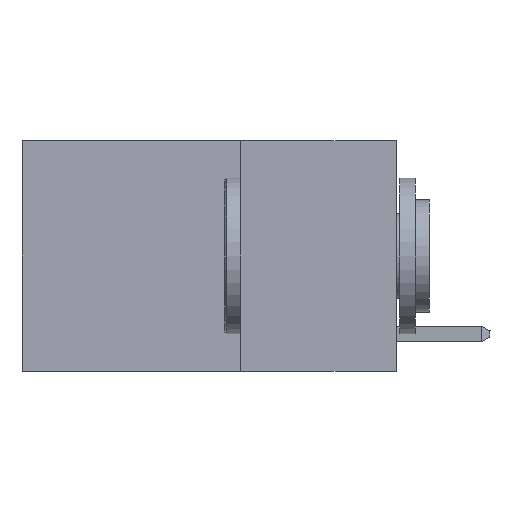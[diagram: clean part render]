
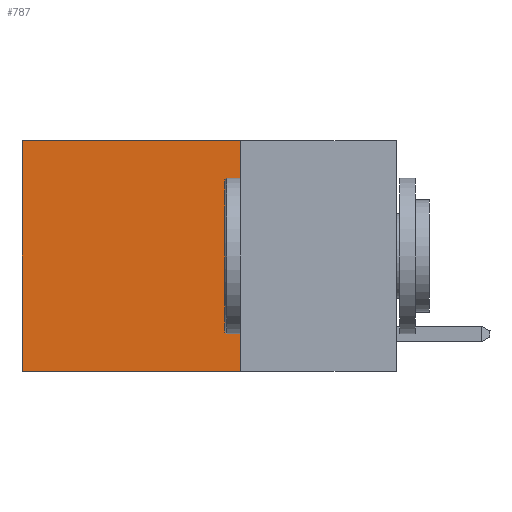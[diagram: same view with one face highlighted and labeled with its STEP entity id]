
A CAD part, left-side view. The second image highlights one B-rep face of the part: STEP entity #787.
In plain terms, the highlighted planar face has unit normal (-1, 0, 0).
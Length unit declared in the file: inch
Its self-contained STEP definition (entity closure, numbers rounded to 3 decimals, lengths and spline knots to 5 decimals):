
#426 = VERTEX_POINT ( 'NONE', #8700 ) ;
#637 = DIRECTION ( 'NONE',  ( 0., 0., -1. ) ) ;
#787 = ADVANCED_FACE ( 'NONE', ( #7513 ), #5920, .F. ) ;
#1073 = EDGE_LOOP ( 'NONE', ( #2785, #2687, #2594, #2554 ) ) ;
#1516 = CARTESIAN_POINT ( 'NONE',  ( 0.2625, 0.6, 0. ) ) ;
#1568 = VERTEX_POINT ( 'NONE', #8690 ) ;
#1801 = VECTOR ( 'NONE', #5940, 39.37008 ) ;
#2161 = VERTEX_POINT ( 'NONE', #1516 ) ;
#2205 = AXIS2_PLACEMENT_3D ( 'NONE', #5118, #5023, #637 ) ;
#2554 = ORIENTED_EDGE ( 'NONE', *, *, #3776, .T. ) ;
#2594 = ORIENTED_EDGE ( 'NONE', *, *, #3153, .F. ) ;
#2649 = VERTEX_POINT ( 'NONE', #7451 ) ;
#2687 = ORIENTED_EDGE ( 'NONE', *, *, #6228, .F. ) ;
#2747 = LINE ( 'NONE', #6149, #1801 ) ;
#2785 = ORIENTED_EDGE ( 'NONE', *, *, #5753, .T. ) ;
#3153 = EDGE_CURVE ( 'NONE', #426, #1568, #8497, .T. ) ;
#3486 = VECTOR ( 'NONE', #3680, 39.37008 ) ;
#3565 = LINE ( 'NONE', #3623, #3486 ) ;
#3623 = CARTESIAN_POINT ( 'NONE',  ( 0.2625, 0.6, 0. ) ) ;
#3626 = CARTESIAN_POINT ( 'NONE',  ( 0.2625, 0.25, 0. ) ) ;
#3680 = DIRECTION ( 'NONE',  ( 0., 0., -1. ) ) ;
#3776 = EDGE_CURVE ( 'NONE', #426, #2161, #5675, .T. ) ;
#4225 = DIRECTION ( 'NONE',  ( 0., 0., -1. ) ) ;
#5023 = DIRECTION ( 'NONE',  ( 1., 0., 0. ) ) ;
#5118 = CARTESIAN_POINT ( 'NONE',  ( 0.2625, 0.25, 0. ) ) ;
#5668 = VECTOR ( 'NONE', #7153, 39.37008 ) ;
#5675 = LINE ( 'NONE', #6978, #5668 ) ;
#5753 = EDGE_CURVE ( 'NONE', #2161, #2649, #3565, .T. ) ;
#5920 = PLANE ( 'NONE',  #2205 ) ;
#5940 = DIRECTION ( 'NONE',  ( 0., 1., 0. ) ) ;
#6149 = CARTESIAN_POINT ( 'NONE',  ( 0.2625, 0.25, -0.37 ) ) ;
#6228 = EDGE_CURVE ( 'NONE', #1568, #2649, #2747, .T. ) ;
#6978 = CARTESIAN_POINT ( 'NONE',  ( 0.2625, 0.25, 0. ) ) ;
#7153 = DIRECTION ( 'NONE',  ( 0., 1., 0. ) ) ;
#7451 = CARTESIAN_POINT ( 'NONE',  ( 0.2625, 0.6, -0.37 ) ) ;
#7513 = FACE_OUTER_BOUND ( 'NONE', #1073, .T. ) ;
#8491 = VECTOR ( 'NONE', #4225, 39.37008 ) ;
#8497 = LINE ( 'NONE', #3626, #8491 ) ;
#8690 = CARTESIAN_POINT ( 'NONE',  ( 0.2625, 0.25, -0.37 ) ) ;
#8700 = CARTESIAN_POINT ( 'NONE',  ( 0.2625, 0.25, 0. ) ) ;
